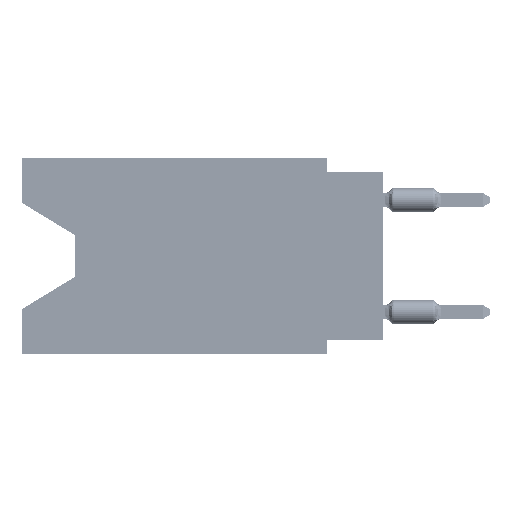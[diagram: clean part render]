
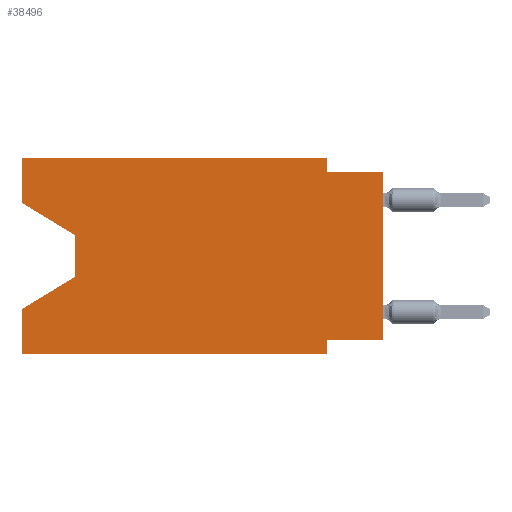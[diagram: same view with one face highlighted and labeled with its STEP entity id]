
A CAD part, left-side view. The second image highlights one B-rep face of the part: STEP entity #38496.
In plain terms, the highlighted planar face has unit normal (-1, 0, 0).
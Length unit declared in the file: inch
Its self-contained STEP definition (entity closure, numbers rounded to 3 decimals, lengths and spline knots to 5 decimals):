
#698 = LINE ( 'NONE', #85675, #89678 ) ;
#4482 = DIRECTION ( 'NONE',  ( 0., 0., -1. ) ) ;
#7360 = CARTESIAN_POINT ( 'NONE',  ( 0., 0., -0.025 ) ) ;
#8830 = ORIENTED_EDGE ( 'NONE', *, *, #44956, .F. ) ;
#11903 = CARTESIAN_POINT ( 'NONE',  ( 0., 0.55, -0.212 ) ) ;
#14539 = DIRECTION ( 'NONE',  ( 0., -1., 0. ) ) ;
#17123 = ORIENTED_EDGE ( 'NONE', *, *, #23097, .F. ) ;
#17206 = VERTEX_POINT ( 'NONE', #89252 ) ;
#17980 = ORIENTED_EDGE ( 'NONE', *, *, #106832, .F. ) ;
#20127 = DIRECTION ( 'NONE',  ( 0., 0., -1. ) ) ;
#23097 = EDGE_CURVE ( 'NONE', #109755, #97035, #111509, .T. ) ;
#23546 = DIRECTION ( 'NONE',  ( 0., 0., 1. ) ) ;
#24961 = EDGE_CURVE ( 'NONE', #107074, #81153, #63626, .T. ) ;
#25068 = CARTESIAN_POINT ( 'NONE',  ( 0., 0.645, -0.35 ) ) ;
#25997 = DIRECTION ( 'NONE',  ( 0., 0., -1. ) ) ;
#26288 = ORIENTED_EDGE ( 'NONE', *, *, #64830, .T. ) ;
#26858 = ORIENTED_EDGE ( 'NONE', *, *, #74053, .F. ) ;
#27411 = DIRECTION ( 'NONE',  ( 0., 0., 1. ) ) ;
#29379 = PLANE ( 'NONE',  #80264 ) ;
#29702 = VECTOR ( 'NONE', #23546, 39.37008 ) ;
#31026 = ORIENTED_EDGE ( 'NONE', *, *, #36325, .T. ) ;
#33385 = VECTOR ( 'NONE', #33430, 39.37008 ) ;
#33430 = DIRECTION ( 'NONE',  ( 0., 0.855, -0.519 ) ) ;
#33758 = CARTESIAN_POINT ( 'NONE',  ( 0., 0.1, -0.35 ) ) ;
#34375 = CARTESIAN_POINT ( 'NONE',  ( 0., 0., -0.325 ) ) ;
#36325 = EDGE_CURVE ( 'NONE', #17206, #114435, #698, .T. ) ;
#36953 = DIRECTION ( 'NONE',  ( 0., 0., 1. ) ) ;
#37852 = ORIENTED_EDGE ( 'NONE', *, *, #115443, .F. ) ;
#38496 = ADVANCED_FACE ( 'NONE', ( #102699 ), #29379, .F. ) ;
#44956 = EDGE_CURVE ( 'NONE', #57602, #49950, #52497, .T. ) ;
#47760 = VERTEX_POINT ( 'NONE', #81404 ) ;
#48139 = DIRECTION ( 'NONE',  ( 0., 0., -1. ) ) ;
#49950 = VERTEX_POINT ( 'NONE', #82973 ) ;
#50990 = VECTOR ( 'NONE', #4482, 39.37008 ) ;
#52293 = ORIENTED_EDGE ( 'NONE', *, *, #81543, .F. ) ;
#52318 = VECTOR ( 'NONE', #81383, 39.37008 ) ;
#52497 = LINE ( 'NONE', #57670, #50990 ) ;
#52820 = VECTOR ( 'NONE', #25997, 39.37008 ) ;
#57116 = VERTEX_POINT ( 'NONE', #11903 ) ;
#57602 = VERTEX_POINT ( 'NONE', #59168 ) ;
#57670 = CARTESIAN_POINT ( 'NONE',  ( 0., 0.1, 0. ) ) ;
#59123 = CARTESIAN_POINT ( 'NONE',  ( 0., 0.55, -0.138 ) ) ;
#59168 = CARTESIAN_POINT ( 'NONE',  ( 0., 0.1, 0. ) ) ;
#59825 = ORIENTED_EDGE ( 'NONE', *, *, #24961, .F. ) ;
#61156 = LINE ( 'NONE', #69788, #33385 ) ;
#62326 = ORIENTED_EDGE ( 'NONE', *, *, #88830, .T. ) ;
#62331 = CARTESIAN_POINT ( 'NONE',  ( 0., 0.645, 0. ) ) ;
#63626 = LINE ( 'NONE', #119103, #118659 ) ;
#63773 = CARTESIAN_POINT ( 'NONE',  ( 0., 0.645, -0.35 ) ) ;
#64830 = EDGE_CURVE ( 'NONE', #109755, #107059, #82856, .T. ) ;
#64971 = VECTOR ( 'NONE', #27411, 39.37008 ) ;
#69788 = CARTESIAN_POINT ( 'NONE',  ( 0., 0.55, -0.212 ) ) ;
#72816 = LINE ( 'NONE', #110409, #52820 ) ;
#72864 = DIRECTION ( 'NONE',  ( 0., 1., 0. ) ) ;
#74053 = EDGE_CURVE ( 'NONE', #47760, #57602, #80779, .T. ) ;
#74443 = VECTOR ( 'NONE', #48139, 39.37008 ) ;
#74529 = CARTESIAN_POINT ( 'NONE',  ( 0., 0.645, 0. ) ) ;
#74616 = DIRECTION ( 'NONE',  ( 0., -0.855, -0.519 ) ) ;
#74788 = CARTESIAN_POINT ( 'NONE',  ( 0., 0.1, -0.325 ) ) ;
#76484 = CARTESIAN_POINT ( 'NONE',  ( 0., 0.55, -0.138 ) ) ;
#78765 = LINE ( 'NONE', #97256, #90991 ) ;
#80264 = AXIS2_PLACEMENT_3D ( 'NONE', #93456, #111344, #20127 ) ;
#80585 = VECTOR ( 'NONE', #14539, 39.37008 ) ;
#80779 = LINE ( 'NONE', #90629, #52318 ) ;
#81031 = CARTESIAN_POINT ( 'NONE',  ( 0., 0., 0. ) ) ;
#81153 = VERTEX_POINT ( 'NONE', #74788 ) ;
#81383 = DIRECTION ( 'NONE',  ( 0., -1., 0. ) ) ;
#81404 = CARTESIAN_POINT ( 'NONE',  ( 0., 0.645, 0. ) ) ;
#81543 = EDGE_CURVE ( 'NONE', #81153, #107059, #72816, .T. ) ;
#82856 = LINE ( 'NONE', #63773, #80585 ) ;
#82962 = EDGE_CURVE ( 'NONE', #114435, #57116, #85717, .T. ) ;
#82973 = CARTESIAN_POINT ( 'NONE',  ( 0., 0.1, -0.025 ) ) ;
#83813 = ORIENTED_EDGE ( 'NONE', *, *, #82962, .T. ) ;
#84544 = EDGE_CURVE ( 'NONE', #57116, #97035, #61156, .T. ) ;
#85195 = VERTEX_POINT ( 'NONE', #7360 ) ;
#85675 = CARTESIAN_POINT ( 'NONE',  ( 0., 0.645, -0.08025 ) ) ;
#85717 = LINE ( 'NONE', #76484, #74443 ) ;
#88087 = ORIENTED_EDGE ( 'NONE', *, *, #84544, .T. ) ;
#88830 = EDGE_CURVE ( 'NONE', #107074, #85195, #100739, .T. ) ;
#89252 = CARTESIAN_POINT ( 'NONE',  ( 0., 0.645, -0.08025 ) ) ;
#89678 = VECTOR ( 'NONE', #74616, 39.37008 ) ;
#90629 = CARTESIAN_POINT ( 'NONE',  ( 0., 0.645, 0. ) ) ;
#90991 = VECTOR ( 'NONE', #105890, 39.37008 ) ;
#91479 = CARTESIAN_POINT ( 'NONE',  ( 0., 0.645, -0.26975 ) ) ;
#92598 = EDGE_LOOP ( 'NONE', ( #31026, #83813, #88087, #17123, #26288, #52293, #59825, #62326, #17980, #8830, #26858, #37852 ) ) ;
#93456 = CARTESIAN_POINT ( 'NONE',  ( 0., 0.645, 0. ) ) ;
#97035 = VERTEX_POINT ( 'NONE', #91479 ) ;
#97256 = CARTESIAN_POINT ( 'NONE',  ( 0., 0., -0.025 ) ) ;
#100739 = LINE ( 'NONE', #81031, #64971 ) ;
#102699 = FACE_OUTER_BOUND ( 'NONE', #92598, .T. ) ;
#105890 = DIRECTION ( 'NONE',  ( 0., -1., 0. ) ) ;
#106832 = EDGE_CURVE ( 'NONE', #49950, #85195, #78765, .T. ) ;
#107059 = VERTEX_POINT ( 'NONE', #33758 ) ;
#107074 = VERTEX_POINT ( 'NONE', #34375 ) ;
#107955 = LINE ( 'NONE', #62331, #29702 ) ;
#109755 = VERTEX_POINT ( 'NONE', #25068 ) ;
#110409 = CARTESIAN_POINT ( 'NONE',  ( 0., 0.1, -0.35 ) ) ;
#111344 = DIRECTION ( 'NONE',  ( 1., 0., 0. ) ) ;
#111509 = LINE ( 'NONE', #74529, #114516 ) ;
#114435 = VERTEX_POINT ( 'NONE', #59123 ) ;
#114516 = VECTOR ( 'NONE', #36953, 39.37008 ) ;
#115443 = EDGE_CURVE ( 'NONE', #17206, #47760, #107955, .T. ) ;
#118659 = VECTOR ( 'NONE', #72864, 39.37008 ) ;
#119103 = CARTESIAN_POINT ( 'NONE',  ( 0., 0., -0.325 ) ) ;
